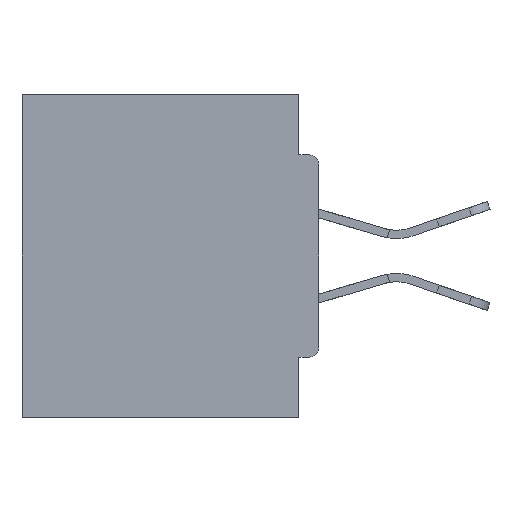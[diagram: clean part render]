
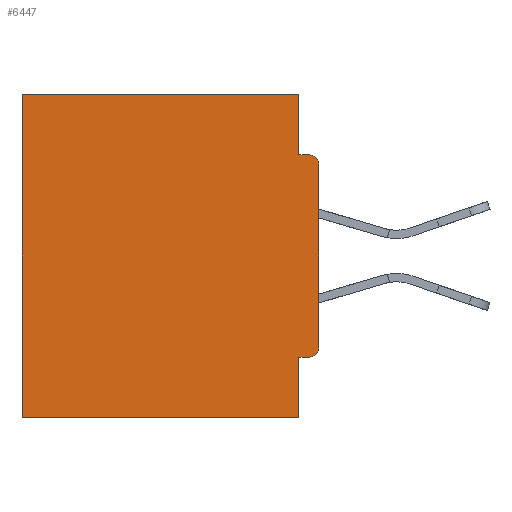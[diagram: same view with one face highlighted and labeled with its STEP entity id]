
A CAD part, left-side view. The second image highlights one B-rep face of the part: STEP entity #6447.
In plain terms, the highlighted planar face has unit normal (-1, 0, 0).
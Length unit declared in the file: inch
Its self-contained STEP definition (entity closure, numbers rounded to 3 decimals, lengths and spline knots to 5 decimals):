
#478 = AXIS2_PLACEMENT_3D ( 'NONE', #6902, #10387, #14001 ) ;
#905 = ORIENTED_EDGE ( 'NONE', *, *, #33017, .T. ) ;
#1017 = ORIENTED_EDGE ( 'NONE', *, *, #32137, .F. ) ;
#1968 = CARTESIAN_POINT ( 'NONE',  ( 0.298, 0.015, -0.3915 ) ) ;
#3314 = LINE ( 'NONE', #17079, #18428 ) ;
#3380 = VECTOR ( 'NONE', #32772, 39.37008 ) ;
#3602 = VERTEX_POINT ( 'NONE', #8911 ) ;
#4559 = CARTESIAN_POINT ( 'NONE',  ( 0.298, 0.015, -0.1085 ) ) ;
#5818 = CARTESIAN_POINT ( 'NONE',  ( 0.298, 0.46, 0. ) ) ;
#6447 = ADVANCED_FACE ( 'NONE', ( #15369 ), #20633, .F. ) ;
#6902 = CARTESIAN_POINT ( 'NONE',  ( 0.298, 0., 0. ) ) ;
#8051 = DIRECTION ( 'NONE',  ( 0., 0., -1. ) ) ;
#8846 = EDGE_CURVE ( 'NONE', #41683, #34025, #29497, .T. ) ;
#8911 = CARTESIAN_POINT ( 'NONE',  ( 0.298, 0.015, -0.0935 ) ) ;
#10387 = DIRECTION ( 'NONE',  ( 1., 0., 0. ) ) ;
#11361 = CARTESIAN_POINT ( 'NONE',  ( 0.298, 0.031, -0.5 ) ) ;
#11995 = CARTESIAN_POINT ( 'NONE',  ( 0.298, 0., -0.3915 ) ) ;
#13616 = LINE ( 'NONE', #35075, #14109 ) ;
#14001 = DIRECTION ( 'NONE',  ( 0., 0., -1. ) ) ;
#14109 = VECTOR ( 'NONE', #24520, 39.37008 ) ;
#14862 = VECTOR ( 'NONE', #32811, 39.37008 ) ;
#14896 = ORIENTED_EDGE ( 'NONE', *, *, #27059, .T. ) ;
#15293 = VECTOR ( 'NONE', #25895, 39.37008 ) ;
#15369 = FACE_OUTER_BOUND ( 'NONE', #21194, .T. ) ;
#15553 = EDGE_CURVE ( 'NONE', #34025, #30789, #31441, .T. ) ;
#16107 = CARTESIAN_POINT ( 'NONE',  ( 0.298, 0., 0. ) ) ;
#16569 = DIRECTION ( 'NONE',  ( 0., 1., 0. ) ) ;
#16755 = VERTEX_POINT ( 'NONE', #23836 ) ;
#16826 = ORIENTED_EDGE ( 'NONE', *, *, #25677, .T. ) ;
#17079 = CARTESIAN_POINT ( 'NONE',  ( 0.298, 0.031, -0.5 ) ) ;
#17223 = VERTEX_POINT ( 'NONE', #11995 ) ;
#17349 = DIRECTION ( 'NONE',  ( 0., 0., -1. ) ) ;
#17870 = EDGE_CURVE ( 'NONE', #19489, #41683, #24848, .T. ) ;
#18284 = VECTOR ( 'NONE', #16569, 39.37008 ) ;
#18428 = VECTOR ( 'NONE', #40843, 39.37008 ) ;
#19489 = VERTEX_POINT ( 'NONE', #32930 ) ;
#19629 = DIRECTION ( 'NONE',  ( 0., 0., -1. ) ) ;
#20633 = PLANE ( 'NONE',  #478 ) ;
#21194 = EDGE_LOOP ( 'NONE', ( #14896, #25343, #28135, #905, #16826, #38849, #29215, #33384, #44643, #1017 ) ) ;
#21751 = LINE ( 'NONE', #25610, #15293 ) ;
#21835 = LINE ( 'NONE', #31574, #42429 ) ;
#23836 = CARTESIAN_POINT ( 'NONE',  ( 0.298, 0.031, -0.0935 ) ) ;
#24110 = VERTEX_POINT ( 'NONE', #42990 ) ;
#24520 = DIRECTION ( 'NONE',  ( 0., -1., 0. ) ) ;
#24623 = CIRCLE ( 'NONE', #28226, 0.015 ) ;
#24848 = LINE ( 'NONE', #44572, #18284 ) ;
#25343 = ORIENTED_EDGE ( 'NONE', *, *, #33659, .F. ) ;
#25610 = CARTESIAN_POINT ( 'NONE',  ( 0.298, 0., 0. ) ) ;
#25677 = EDGE_CURVE ( 'NONE', #40549, #30789, #21835, .T. ) ;
#25895 = DIRECTION ( 'NONE',  ( 0., 1., 0. ) ) ;
#26095 = VECTOR ( 'NONE', #30011, 39.37008 ) ;
#27059 = EDGE_CURVE ( 'NONE', #24110, #3602, #43349, .T. ) ;
#28135 = ORIENTED_EDGE ( 'NONE', *, *, #33547, .F. ) ;
#28226 = AXIS2_PLACEMENT_3D ( 'NONE', #1968, #33417, #19629 ) ;
#28781 = DIRECTION ( 'NONE',  ( -1., 0., 0. ) ) ;
#29215 = ORIENTED_EDGE ( 'NONE', *, *, #8846, .F. ) ;
#29497 = LINE ( 'NONE', #11361, #14862 ) ;
#30011 = DIRECTION ( 'NONE',  ( 0., 1., 0. ) ) ;
#30084 = VERTEX_POINT ( 'NONE', #36080 ) ;
#30789 = VERTEX_POINT ( 'NONE', #41016 ) ;
#31005 = EDGE_CURVE ( 'NONE', #19489, #17223, #24623, .T. ) ;
#31098 = CARTESIAN_POINT ( 'NONE',  ( 0.298, 0.031, -0.5 ) ) ;
#31441 = LINE ( 'NONE', #43766, #26095 ) ;
#31574 = CARTESIAN_POINT ( 'NONE',  ( 0.298, 0.46, 0. ) ) ;
#32137 = EDGE_CURVE ( 'NONE', #24110, #17223, #34771, .T. ) ;
#32772 = DIRECTION ( 'NONE',  ( 0., 0., -1. ) ) ;
#32811 = DIRECTION ( 'NONE',  ( 0., 0., -1. ) ) ;
#32930 = CARTESIAN_POINT ( 'NONE',  ( 0.298, 0.015, -0.4065 ) ) ;
#33017 = EDGE_CURVE ( 'NONE', #30084, #40549, #21751, .T. ) ;
#33384 = ORIENTED_EDGE ( 'NONE', *, *, #17870, .F. ) ;
#33417 = DIRECTION ( 'NONE',  ( -1., 0., 0. ) ) ;
#33547 = EDGE_CURVE ( 'NONE', #30084, #16755, #3314, .T. ) ;
#33659 = EDGE_CURVE ( 'NONE', #16755, #3602, #13616, .T. ) ;
#34025 = VERTEX_POINT ( 'NONE', #31098 ) ;
#34247 = AXIS2_PLACEMENT_3D ( 'NONE', #4559, #28781, #8051 ) ;
#34771 = LINE ( 'NONE', #16107, #3380 ) ;
#35075 = CARTESIAN_POINT ( 'NONE',  ( 0.298, 0., -0.0935 ) ) ;
#36080 = CARTESIAN_POINT ( 'NONE',  ( 0.298, 0.031, 0. ) ) ;
#38849 = ORIENTED_EDGE ( 'NONE', *, *, #15553, .F. ) ;
#40549 = VERTEX_POINT ( 'NONE', #5818 ) ;
#40843 = DIRECTION ( 'NONE',  ( 0., 0., -1. ) ) ;
#41016 = CARTESIAN_POINT ( 'NONE',  ( 0.298, 0.46, -0.5 ) ) ;
#41683 = VERTEX_POINT ( 'NONE', #41898 ) ;
#41898 = CARTESIAN_POINT ( 'NONE',  ( 0.298, 0.031, -0.4065 ) ) ;
#42429 = VECTOR ( 'NONE', #17349, 39.37008 ) ;
#42990 = CARTESIAN_POINT ( 'NONE',  ( 0.298, 0., -0.1085 ) ) ;
#43349 = CIRCLE ( 'NONE', #34247, 0.015 ) ;
#43766 = CARTESIAN_POINT ( 'NONE',  ( 0.298, 0., -0.5 ) ) ;
#44572 = CARTESIAN_POINT ( 'NONE',  ( 0.298, 0., -0.4065 ) ) ;
#44643 = ORIENTED_EDGE ( 'NONE', *, *, #31005, .T. ) ;
